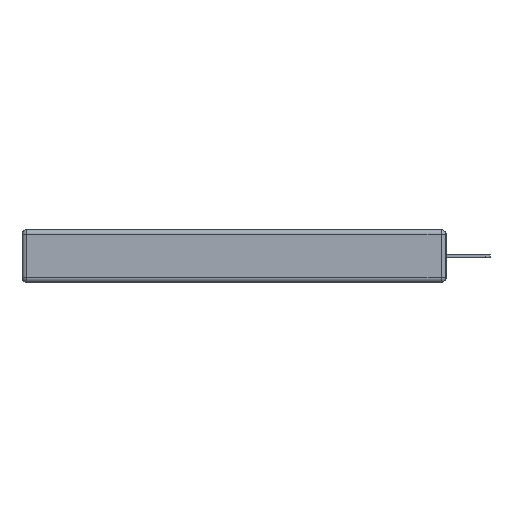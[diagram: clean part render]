
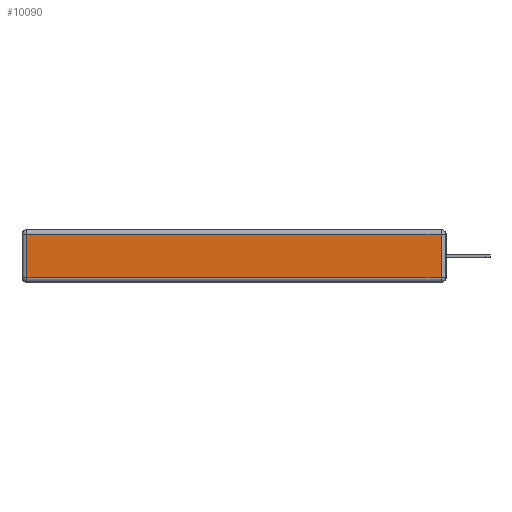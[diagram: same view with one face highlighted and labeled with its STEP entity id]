
A CAD part, left-side view. The second image highlights one B-rep face of the part: STEP entity #10090.
In plain terms, the highlighted planar face has unit normal (-1, 0, 0).
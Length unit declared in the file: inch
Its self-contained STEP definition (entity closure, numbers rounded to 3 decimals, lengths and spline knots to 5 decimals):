
#1811 = CARTESIAN_POINT ( 'NONE',  ( 0., 0.03, -0.343 ) ) ;
#2528 = DIRECTION ( 'NONE',  ( 0., 1., 0. ) ) ;
#2567 = CARTESIAN_POINT ( 'NONE',  ( 0., 0., -0.343 ) ) ;
#5185 = AXIS2_PLACEMENT_3D ( 'NONE', #2567, #7007, #20430 ) ;
#5225 = CARTESIAN_POINT ( 'NONE',  ( 0., 2.72, -0.313 ) ) ;
#5264 = VECTOR ( 'NONE', #22361, 39.37008 ) ;
#6368 = DIRECTION ( 'NONE',  ( 0., -1., 0. ) ) ;
#6453 = LINE ( 'NONE', #21913, #21026 ) ;
#6758 = EDGE_CURVE ( 'NONE', #21347, #24167, #12164, .T. ) ;
#7007 = DIRECTION ( 'NONE',  ( -1., 0., 0. ) ) ;
#7790 = CARTESIAN_POINT ( 'NONE',  ( 0., 0.03, -0.03 ) ) ;
#7801 = VERTEX_POINT ( 'NONE', #15502 ) ;
#8745 = EDGE_CURVE ( 'NONE', #11127, #7801, #6453, .T. ) ;
#9654 = ORIENTED_EDGE ( 'NONE', *, *, #20001, .T. ) ;
#10090 = ADVANCED_FACE ( 'NONE', ( #24523 ), #20055, .T. ) ;
#10740 = CARTESIAN_POINT ( 'NONE',  ( 0., 0., -0.313 ) ) ;
#11127 = VERTEX_POINT ( 'NONE', #7790 ) ;
#12164 = LINE ( 'NONE', #10740, #24917 ) ;
#12434 = CARTESIAN_POINT ( 'NONE',  ( 0., 2.72, -0.343 ) ) ;
#13040 = EDGE_CURVE ( 'NONE', #24167, #11127, #23271, .T. ) ;
#15085 = VECTOR ( 'NONE', #17638, 39.37008 ) ;
#15502 = CARTESIAN_POINT ( 'NONE',  ( 0., 2.72, -0.03 ) ) ;
#16357 = LINE ( 'NONE', #12434, #5264 ) ;
#17100 = ORIENTED_EDGE ( 'NONE', *, *, #6758, .T. ) ;
#17638 = DIRECTION ( 'NONE',  ( 0., 0., 1. ) ) ;
#18431 = EDGE_LOOP ( 'NONE', ( #17100, #22066, #21495, #9654 ) ) ;
#20001 = EDGE_CURVE ( 'NONE', #7801, #21347, #16357, .T. ) ;
#20055 = PLANE ( 'NONE',  #5185 ) ;
#20430 = DIRECTION ( 'NONE',  ( 0., 0., 1. ) ) ;
#21026 = VECTOR ( 'NONE', #2528, 39.37008 ) ;
#21347 = VERTEX_POINT ( 'NONE', #5225 ) ;
#21495 = ORIENTED_EDGE ( 'NONE', *, *, #8745, .T. ) ;
#21913 = CARTESIAN_POINT ( 'NONE',  ( 0., 2.75, -0.03 ) ) ;
#22066 = ORIENTED_EDGE ( 'NONE', *, *, #13040, .T. ) ;
#22361 = DIRECTION ( 'NONE',  ( 0., 0., -1. ) ) ;
#23271 = LINE ( 'NONE', #1811, #15085 ) ;
#23507 = CARTESIAN_POINT ( 'NONE',  ( 0., 0.03, -0.313 ) ) ;
#24167 = VERTEX_POINT ( 'NONE', #23507 ) ;
#24523 = FACE_OUTER_BOUND ( 'NONE', #18431, .T. ) ;
#24917 = VECTOR ( 'NONE', #6368, 39.37008 ) ;
